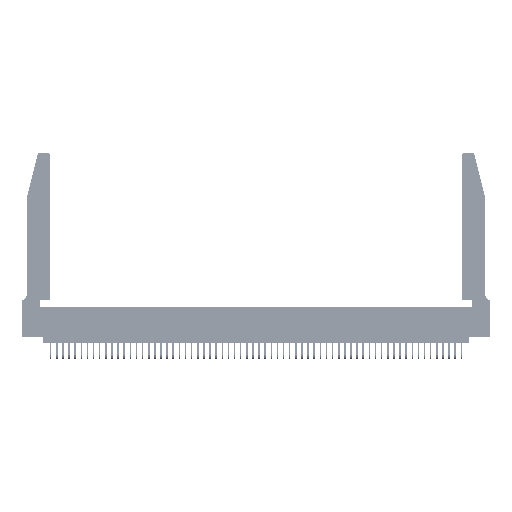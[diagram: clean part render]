
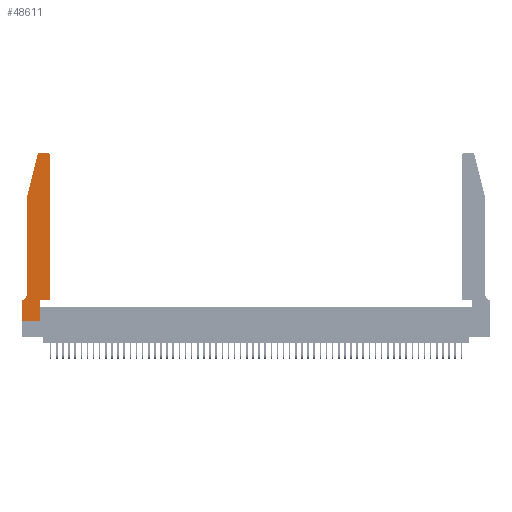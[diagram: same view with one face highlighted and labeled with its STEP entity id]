
A CAD part, top view. The second image highlights one B-rep face of the part: STEP entity #48611.
In plain terms, the highlighted planar face has unit normal (0, 0, 1).
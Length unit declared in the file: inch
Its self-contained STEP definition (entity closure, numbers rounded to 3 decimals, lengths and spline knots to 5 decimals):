
#860 = VERTEX_POINT ( 'NONE', #36091 ) ;
#3121 = EDGE_CURVE ( 'NONE', #7286, #860, #15807, .T. ) ;
#4218 = CARTESIAN_POINT ( 'NONE',  ( 0., 0., 0.37 ) ) ;
#4609 = CARTESIAN_POINT ( 'NONE',  ( 0.2865, 0.35, 0.37 ) ) ;
#4857 = LINE ( 'NONE', #10162, #26646 ) ;
#4975 = ORIENTED_EDGE ( 'NONE', *, *, #20801, .T. ) ;
#5784 = VECTOR ( 'NONE', #45645, 39.37008 ) ;
#5983 = DIRECTION ( 'NONE',  ( 0., 0., 1. ) ) ;
#6680 = CARTESIAN_POINT ( 'NONE',  ( 0.0755, 2., 0.37 ) ) ;
#7286 = VERTEX_POINT ( 'NONE', #31074 ) ;
#7373 = EDGE_CURVE ( 'NONE', #860, #50373, #52322, .T. ) ;
#10077 = VECTOR ( 'NONE', #19800, 39.37008 ) ;
#10162 = CARTESIAN_POINT ( 'NONE',  ( 0.4505, 0.35, 0.37 ) ) ;
#11049 = ORIENTED_EDGE ( 'NONE', *, *, #3121, .T. ) ;
#12530 = DIRECTION ( 'NONE',  ( 1., 0., 0. ) ) ;
#14410 = CARTESIAN_POINT ( 'NONE',  ( 0.4505, 2.72, 0.37 ) ) ;
#14512 = ORIENTED_EDGE ( 'NONE', *, *, #23400, .T. ) ;
#15229 = ORIENTED_EDGE ( 'NONE', *, *, #32519, .T. ) ;
#15258 = CARTESIAN_POINT ( 'NONE',  ( 0., 0.35, 0.37 ) ) ;
#15807 = LINE ( 'NONE', #17991, #37553 ) ;
#16097 = LINE ( 'NONE', #39644, #39219 ) ;
#16518 = CARTESIAN_POINT ( 'NONE',  ( 0.0055, 0.42, 0.37 ) ) ;
#17398 = LINE ( 'NONE', #19666, #5784 ) ;
#17606 = LINE ( 'NONE', #47735, #50818 ) ;
#17825 = CARTESIAN_POINT ( 'NONE',  ( 0.4205, 2.72, 0.37 ) ) ;
#17877 = CARTESIAN_POINT ( 'NONE',  ( 0.0055, 0.35, 0.37 ) ) ;
#17975 = AXIS2_PLACEMENT_3D ( 'NONE', #38405, #38591, #12530 ) ;
#17991 = CARTESIAN_POINT ( 'NONE',  ( 0.2605, 2.75, 0.37 ) ) ;
#18418 = LINE ( 'NONE', #35785, #40173 ) ;
#19534 = EDGE_CURVE ( 'NONE', #50715, #52664, #20483, .T. ) ;
#19666 = CARTESIAN_POINT ( 'NONE',  ( 0., 0., 0.37 ) ) ;
#19800 = DIRECTION ( 'NONE',  ( 0., 1., 0. ) ) ;
#20483 = LINE ( 'NONE', #6680, #42215 ) ;
#20801 = EDGE_CURVE ( 'NONE', #52340, #46659, #44741, .T. ) ;
#20855 = DIRECTION ( 'NONE',  ( -1., 0., 0. ) ) ;
#21428 = VERTEX_POINT ( 'NONE', #28471 ) ;
#22184 = DIRECTION ( 'NONE',  ( 1., 0., 0. ) ) ;
#22353 = DIRECTION ( 'NONE',  ( 1., 0., 0. ) ) ;
#22696 = ORIENTED_EDGE ( 'NONE', *, *, #46634, .T. ) ;
#22963 = CARTESIAN_POINT ( 'NONE',  ( 0.2865, 0.35, 0.37 ) ) ;
#23206 = VERTEX_POINT ( 'NONE', #17877 ) ;
#23400 = EDGE_CURVE ( 'NONE', #25934, #41560, #17398, .T. ) ;
#23650 = DIRECTION ( 'NONE',  ( -1., 0., 0. ) ) ;
#24008 = CARTESIAN_POINT ( 'NONE',  ( 0.4505, 0.35, 0.37 ) ) ;
#24213 = AXIS2_PLACEMENT_3D ( 'NONE', #17825, #48149, #22184 ) ;
#24448 = CARTESIAN_POINT ( 'NONE',  ( 0.0755, 2., 0.37 ) ) ;
#24721 = ORIENTED_EDGE ( 'NONE', *, *, #33191, .T. ) ;
#24777 = ORIENTED_EDGE ( 'NONE', *, *, #50438, .T. ) ;
#24888 = EDGE_CURVE ( 'NONE', #52664, #23206, #40379, .T. ) ;
#25934 = VERTEX_POINT ( 'NONE', #15258 ) ;
#26236 = VECTOR ( 'NONE', #44568, 39.37008 ) ;
#26646 = VECTOR ( 'NONE', #40598, 39.37008 ) ;
#26720 = ORIENTED_EDGE ( 'NONE', *, *, #50949, .T. ) ;
#27560 = LINE ( 'NONE', #22963, #26236 ) ;
#28471 = CARTESIAN_POINT ( 'NONE',  ( 0.2865, 0., 0.37 ) ) ;
#29402 = FACE_OUTER_BOUND ( 'NONE', #52341, .T. ) ;
#30768 = ORIENTED_EDGE ( 'NONE', *, *, #19534, .T. ) ;
#31074 = CARTESIAN_POINT ( 'NONE',  ( 0.4205, 2.75, 0.37 ) ) ;
#32020 = CARTESIAN_POINT ( 'NONE',  ( 0.284, 2.72, 0.37 ) ) ;
#32519 = EDGE_CURVE ( 'NONE', #47425, #52340, #4857, .T. ) ;
#33191 = EDGE_CURVE ( 'NONE', #23206, #25934, #18418, .T. ) ;
#34199 = PLANE ( 'NONE',  #17975 ) ;
#35405 = AXIS2_PLACEMENT_3D ( 'NONE', #16518, #46818, #20855 ) ;
#35785 = CARTESIAN_POINT ( 'NONE',  ( 0.0755, 0.35, 0.37 ) ) ;
#36091 = CARTESIAN_POINT ( 'NONE',  ( 0.284, 2.75, 0.37 ) ) ;
#36408 = DIRECTION ( 'NONE',  ( 1., 0., 0. ) ) ;
#37553 = VECTOR ( 'NONE', #52648, 39.37008 ) ;
#38405 = CARTESIAN_POINT ( 'NONE',  ( 0., 0.35, 0.37 ) ) ;
#38591 = DIRECTION ( 'NONE',  ( 0., 0., 1. ) ) ;
#38929 = CARTESIAN_POINT ( 'NONE',  ( 0.25487, 2.72718, 0.37 ) ) ;
#39219 = VECTOR ( 'NONE', #22353, 39.37008 ) ;
#39644 = CARTESIAN_POINT ( 'NONE',  ( 0., 0., 0.37 ) ) ;
#40173 = VECTOR ( 'NONE', #23650, 39.37008 ) ;
#40347 = ORIENTED_EDGE ( 'NONE', *, *, #41670, .T. ) ;
#40379 = CIRCLE ( 'NONE', #35405, 0.07 ) ;
#40598 = DIRECTION ( 'NONE',  ( 1., 0., 0. ) ) ;
#41560 = VERTEX_POINT ( 'NONE', #4218 ) ;
#41670 = EDGE_CURVE ( 'NONE', #41560, #21428, #16097, .T. ) ;
#42104 = CIRCLE ( 'NONE', #24213, 0.03 ) ;
#42215 = VECTOR ( 'NONE', #45772, 39.37008 ) ;
#43689 = ORIENTED_EDGE ( 'NONE', *, *, #24888, .T. ) ;
#44543 = CARTESIAN_POINT ( 'NONE',  ( 0.4505, 0.35, 0.37 ) ) ;
#44568 = DIRECTION ( 'NONE',  ( 0., 1., 0. ) ) ;
#44741 = LINE ( 'NONE', #24008, #10077 ) ;
#45645 = DIRECTION ( 'NONE',  ( 0., -1., 0. ) ) ;
#45772 = DIRECTION ( 'NONE',  ( 0., -1., 0. ) ) ;
#46634 = EDGE_CURVE ( 'NONE', #21428, #47425, #27560, .T. ) ;
#46659 = VERTEX_POINT ( 'NONE', #14410 ) ;
#46818 = DIRECTION ( 'NONE',  ( 0., 0., -1. ) ) ;
#47425 = VERTEX_POINT ( 'NONE', #4609 ) ;
#47735 = CARTESIAN_POINT ( 'NONE',  ( 0.0755, 2., 0.37 ) ) ;
#48149 = DIRECTION ( 'NONE',  ( 0., 0., 1. ) ) ;
#48421 = ORIENTED_EDGE ( 'NONE', *, *, #7373, .T. ) ;
#48611 = ADVANCED_FACE ( 'NONE', ( #29402 ), #34199, .T. ) ;
#50373 = VERTEX_POINT ( 'NONE', #38929 ) ;
#50438 = EDGE_CURVE ( 'NONE', #46659, #7286, #42104, .T. ) ;
#50715 = VERTEX_POINT ( 'NONE', #24448 ) ;
#50800 = AXIS2_PLACEMENT_3D ( 'NONE', #32020, #5983, #36408 ) ;
#50818 = VECTOR ( 'NONE', #56416, 39.37008 ) ;
#50949 = EDGE_CURVE ( 'NONE', #50373, #50715, #17606, .T. ) ;
#52322 = CIRCLE ( 'NONE', #50800, 0.03 ) ;
#52340 = VERTEX_POINT ( 'NONE', #44543 ) ;
#52341 = EDGE_LOOP ( 'NONE', ( #11049, #48421, #26720, #30768, #43689, #24721, #14512, #40347, #22696, #15229, #4975, #24777 ) ) ;
#52648 = DIRECTION ( 'NONE',  ( -1., 0., 0. ) ) ;
#52664 = VERTEX_POINT ( 'NONE', #55661 ) ;
#55661 = CARTESIAN_POINT ( 'NONE',  ( 0.0755, 0.42, 0.37 ) ) ;
#56416 = DIRECTION ( 'NONE',  ( -0.239, -0.971, 0. ) ) ;
